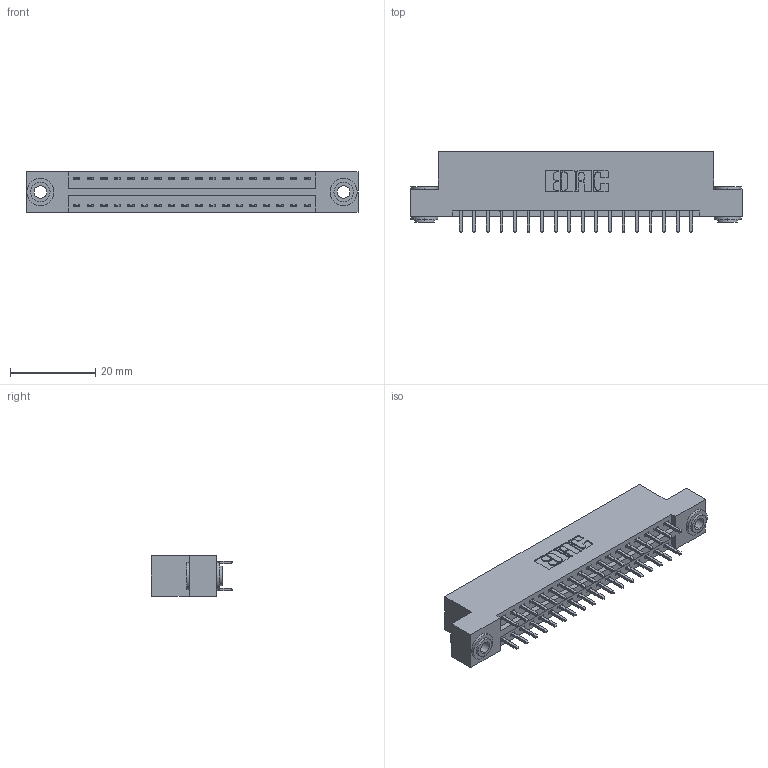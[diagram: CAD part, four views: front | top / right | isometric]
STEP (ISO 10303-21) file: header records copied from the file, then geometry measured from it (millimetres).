
FILE_DESCRIPTION (( 'STEP AP203' ), '1' );
FILE_NAME ('346-036-521-203.STEP', '2022-05-19T21:06:05', ( '' ), ( '' ), 'SwSTEP 2.0', 'SolidWorks 2020', '' );
FILE_SCHEMA (( 'CONFIG_CONTROL_DESIGN' ));
Length unit declared in the file: inch
Products named in the file (4): 346 Part_Flush Mounting Lugs - 0.156 Dia-TH; 345-250-002_345-250-002-102; 345-292-001_345-293-121; 346-036-521-203
Assembly tree (39 placements, depth 2):
  346-036-521-203
    346 Part_Flush Mounting Lugs - 0.156 Dia-TH
    345-292-001_345-293-121  x36
    345-250-002_345-250-002-102  x2
Bounding box: 77.72 x 19.05 x 9.4 mm (x, y, z)
Volume: 7379.3 mm3; surface area: 9915.8 mm2
Topology: 39 solids, 39 shells, 2046 faces, 6021 edges, 3962 vertices
Faces by surface type: plane 1360, cylinder 678, cone 8
Entity records: 16062 total; most frequent: CARTESIAN_POINT 2661, ORIENTED_EDGE 2586, DIRECTION 2427, EDGE_CURVE 1293, VECTOR 1065, LINE 1065, VERTEX_POINT 858, AXIS2_PLACEMENT_3D 681
